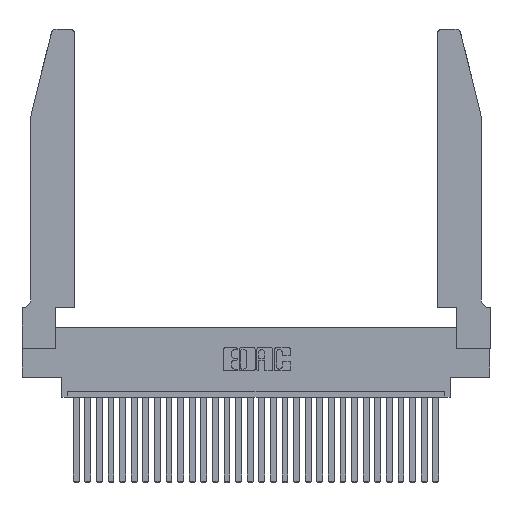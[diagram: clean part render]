
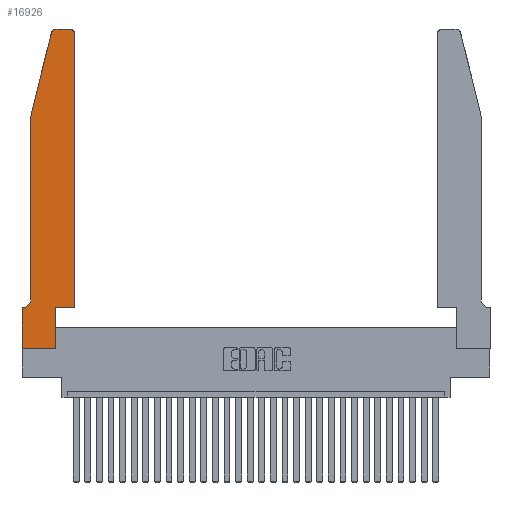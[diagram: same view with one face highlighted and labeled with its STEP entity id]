
A CAD part, top view. The second image highlights one B-rep face of the part: STEP entity #16926.
In plain terms, the highlighted planar face has unit normal (0, 0, 1).
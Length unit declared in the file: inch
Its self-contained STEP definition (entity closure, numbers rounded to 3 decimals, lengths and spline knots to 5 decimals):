
#74 = VERTEX_POINT ( 'NONE', #4018 ) ;
#117 = CARTESIAN_POINT ( 'NONE',  ( 0.0055, 0.42, 0.37 ) ) ;
#491 = VERTEX_POINT ( 'NONE', #22714 ) ;
#722 = VECTOR ( 'NONE', #3054, 39.37008 ) ;
#754 = ORIENTED_EDGE ( 'NONE', *, *, #18174, .T. ) ;
#913 = ORIENTED_EDGE ( 'NONE', *, *, #1210, .T. ) ;
#1210 = EDGE_CURVE ( 'NONE', #74, #4891, #10021, .T. ) ;
#1626 = VERTEX_POINT ( 'NONE', #24817 ) ;
#1657 = CARTESIAN_POINT ( 'NONE',  ( 0.0055, 0.35, 0.37 ) ) ;
#1904 = ORIENTED_EDGE ( 'NONE', *, *, #5158, .T. ) ;
#2153 = EDGE_CURVE ( 'NONE', #1626, #27226, #6734, .T. ) ;
#2263 = CARTESIAN_POINT ( 'NONE',  ( 0., 0.35, 0.37 ) ) ;
#2437 = DIRECTION ( 'NONE',  ( -1., 0., 0. ) ) ;
#3054 = DIRECTION ( 'NONE',  ( 1., 0., 0. ) ) ;
#3278 = ORIENTED_EDGE ( 'NONE', *, *, #27477, .T. ) ;
#3575 = LINE ( 'NONE', #16944, #27608 ) ;
#4018 = CARTESIAN_POINT ( 'NONE',  ( 0.2865, 0., 0.37 ) ) ;
#4104 = CARTESIAN_POINT ( 'NONE',  ( 0.2605, 2.75, 0.37 ) ) ;
#4891 = VERTEX_POINT ( 'NONE', #5617 ) ;
#4949 = VERTEX_POINT ( 'NONE', #1657 ) ;
#5022 = CARTESIAN_POINT ( 'NONE',  ( 0.4205, 2.72, 0.37 ) ) ;
#5158 = EDGE_CURVE ( 'NONE', #19822, #28687, #26582, .T. ) ;
#5322 = CARTESIAN_POINT ( 'NONE',  ( 0.4505, 0.35, 0.37 ) ) ;
#5617 = CARTESIAN_POINT ( 'NONE',  ( 0.2865, 0.35, 0.37 ) ) ;
#6045 = CARTESIAN_POINT ( 'NONE',  ( 0.4505, 0.35, 0.37 ) ) ;
#6395 = ORIENTED_EDGE ( 'NONE', *, *, #23504, .T. ) ;
#6562 = AXIS2_PLACEMENT_3D ( 'NONE', #17410, #14989, #19768 ) ;
#6734 = LINE ( 'NONE', #4104, #9277 ) ;
#8112 = EDGE_CURVE ( 'NONE', #27768, #10790, #26012, .T. ) ;
#9277 = VECTOR ( 'NONE', #10631, 39.37008 ) ;
#9297 = AXIS2_PLACEMENT_3D ( 'NONE', #5022, #12424, #21370 ) ;
#9962 = CARTESIAN_POINT ( 'NONE',  ( 0.2865, 0.35, 0.37 ) ) ;
#10021 = LINE ( 'NONE', #9962, #19460 ) ;
#10106 = LINE ( 'NONE', #26568, #23234 ) ;
#10469 = LINE ( 'NONE', #29779, #29400 ) ;
#10552 = VECTOR ( 'NONE', #24444, 39.37008 ) ;
#10587 = LINE ( 'NONE', #5322, #24423 ) ;
#10631 = DIRECTION ( 'NONE',  ( -1., 0., 0. ) ) ;
#10790 = VERTEX_POINT ( 'NONE', #15962 ) ;
#10944 = CARTESIAN_POINT ( 'NONE',  ( 0.284, 2.72, 0.37 ) ) ;
#11166 = ORIENTED_EDGE ( 'NONE', *, *, #16191, .T. ) ;
#11671 = VERTEX_POINT ( 'NONE', #2263 ) ;
#11686 = DIRECTION ( 'NONE',  ( 0., 1., 0. ) ) ;
#12198 = CIRCLE ( 'NONE', #9297, 0.03 ) ;
#12293 = DIRECTION ( 'NONE',  ( 0., 1., 0. ) ) ;
#12424 = DIRECTION ( 'NONE',  ( 0., 0., 1. ) ) ;
#12505 = FACE_OUTER_BOUND ( 'NONE', #22870, .T. ) ;
#12520 = VECTOR ( 'NONE', #11686, 39.37008 ) ;
#12605 = DIRECTION ( 'NONE',  ( -0.239, -0.971, 0. ) ) ;
#12919 = CARTESIAN_POINT ( 'NONE',  ( 0.0755, 2., 0.37 ) ) ;
#14660 = AXIS2_PLACEMENT_3D ( 'NONE', #117, #16523, #2437 ) ;
#14989 = DIRECTION ( 'NONE',  ( 0., 0., 1. ) ) ;
#15557 = EDGE_CURVE ( 'NONE', #491, #74, #15588, .T. ) ;
#15588 = LINE ( 'NONE', #24128, #722 ) ;
#15674 = ORIENTED_EDGE ( 'NONE', *, *, #20851, .T. ) ;
#15962 = CARTESIAN_POINT ( 'NONE',  ( 0.4505, 2.72, 0.37 ) ) ;
#16123 = ORIENTED_EDGE ( 'NONE', *, *, #15557, .T. ) ;
#16191 = EDGE_CURVE ( 'NONE', #11671, #491, #3575, .T. ) ;
#16523 = DIRECTION ( 'NONE',  ( 0., 0., -1. ) ) ;
#16920 = CARTESIAN_POINT ( 'NONE',  ( 0.284, 2.75, 0.37 ) ) ;
#16926 = ADVANCED_FACE ( 'NONE', ( #12505 ), #24380, .T. ) ;
#16944 = CARTESIAN_POINT ( 'NONE',  ( 0., 0., 0.37 ) ) ;
#17410 = CARTESIAN_POINT ( 'NONE',  ( 0., 0.35, 0.37 ) ) ;
#17646 = CIRCLE ( 'NONE', #28055, 0.03 ) ;
#17805 = DIRECTION ( 'NONE',  ( 1., 0., 0. ) ) ;
#18174 = EDGE_CURVE ( 'NONE', #4891, #27768, #10587, .T. ) ;
#19460 = VECTOR ( 'NONE', #12293, 39.37008 ) ;
#19564 = ORIENTED_EDGE ( 'NONE', *, *, #8112, .T. ) ;
#19768 = DIRECTION ( 'NONE',  ( 1., 0., 0. ) ) ;
#19822 = VERTEX_POINT ( 'NONE', #28126 ) ;
#20368 = DIRECTION ( 'NONE',  ( 0., 0., 1. ) ) ;
#20851 = EDGE_CURVE ( 'NONE', #4949, #11671, #10469, .T. ) ;
#21200 = CIRCLE ( 'NONE', #14660, 0.07 ) ;
#21370 = DIRECTION ( 'NONE',  ( 1., 0., 0. ) ) ;
#21545 = ORIENTED_EDGE ( 'NONE', *, *, #26577, .T. ) ;
#21982 = DIRECTION ( 'NONE',  ( 0., -1., 0. ) ) ;
#22319 = CARTESIAN_POINT ( 'NONE',  ( 0.25487, 2.72718, 0.37 ) ) ;
#22714 = CARTESIAN_POINT ( 'NONE',  ( 0., 0., 0.37 ) ) ;
#22870 = EDGE_LOOP ( 'NONE', ( #23241, #3278, #21545, #1904, #6395, #15674, #11166, #16123, #913, #754, #19564, #26602 ) ) ;
#23234 = VECTOR ( 'NONE', #12605, 39.37008 ) ;
#23241 = ORIENTED_EDGE ( 'NONE', *, *, #2153, .T. ) ;
#23504 = EDGE_CURVE ( 'NONE', #28687, #4949, #21200, .T. ) ;
#23517 = CARTESIAN_POINT ( 'NONE',  ( 0.4505, 0.35, 0.37 ) ) ;
#23817 = CARTESIAN_POINT ( 'NONE',  ( 0.0755, 0.42, 0.37 ) ) ;
#24128 = CARTESIAN_POINT ( 'NONE',  ( 0., 0., 0.37 ) ) ;
#24380 = PLANE ( 'NONE',  #6562 ) ;
#24423 = VECTOR ( 'NONE', #28439, 39.37008 ) ;
#24444 = DIRECTION ( 'NONE',  ( 0., -1., 0. ) ) ;
#24817 = CARTESIAN_POINT ( 'NONE',  ( 0.4205, 2.75, 0.37 ) ) ;
#25500 = DIRECTION ( 'NONE',  ( -1., 0., 0. ) ) ;
#26012 = LINE ( 'NONE', #23517, #12520 ) ;
#26568 = CARTESIAN_POINT ( 'NONE',  ( 0.0755, 2., 0.37 ) ) ;
#26577 = EDGE_CURVE ( 'NONE', #29887, #19822, #10106, .T. ) ;
#26582 = LINE ( 'NONE', #12919, #10552 ) ;
#26602 = ORIENTED_EDGE ( 'NONE', *, *, #28170, .T. ) ;
#27226 = VERTEX_POINT ( 'NONE', #16920 ) ;
#27477 = EDGE_CURVE ( 'NONE', #27226, #29887, #17646, .T. ) ;
#27608 = VECTOR ( 'NONE', #21982, 39.37008 ) ;
#27768 = VERTEX_POINT ( 'NONE', #6045 ) ;
#28055 = AXIS2_PLACEMENT_3D ( 'NONE', #10944, #20368, #17805 ) ;
#28126 = CARTESIAN_POINT ( 'NONE',  ( 0.0755, 2., 0.37 ) ) ;
#28170 = EDGE_CURVE ( 'NONE', #10790, #1626, #12198, .T. ) ;
#28439 = DIRECTION ( 'NONE',  ( 1., 0., 0. ) ) ;
#28687 = VERTEX_POINT ( 'NONE', #23817 ) ;
#29400 = VECTOR ( 'NONE', #25500, 39.37008 ) ;
#29779 = CARTESIAN_POINT ( 'NONE',  ( 0.0755, 0.35, 0.37 ) ) ;
#29887 = VERTEX_POINT ( 'NONE', #22319 ) ;
